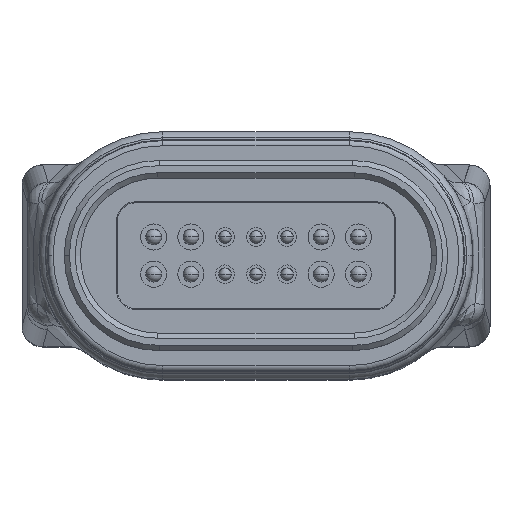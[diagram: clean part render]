
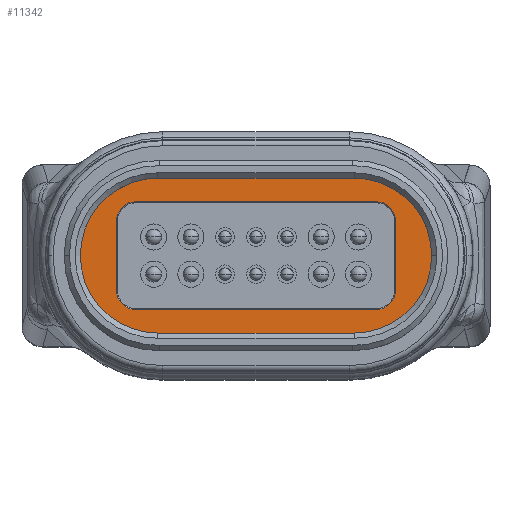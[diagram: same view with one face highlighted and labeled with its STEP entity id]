
A CAD part, top view. The second image highlights one B-rep face of the part: STEP entity #11342.
In plain terms, the highlighted planar face has unit normal (0, 0, 1).
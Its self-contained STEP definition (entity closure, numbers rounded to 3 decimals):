
#337 = ORIENTED_EDGE ( 'NONE', *, *, #929, .T. ) ;
#457 = DIRECTION ( 'NONE',  ( 1., 0., 0. ) ) ;
#584 = DIRECTION ( 'NONE',  ( 1., 0., 0. ) ) ;
#798 = DIRECTION ( 'NONE',  ( -1., 0., 0. ) ) ;
#880 = CIRCLE ( 'NONE', #7388, 0.9 ) ;
#891 = EDGE_CURVE ( 'NONE', #6130, #6328, #986, .T. ) ;
#905 = DIRECTION ( 'NONE',  ( 1., 0., 0. ) ) ;
#929 = EDGE_CURVE ( 'NONE', #8517, #8174, #2845, .T. ) ;
#960 = CARTESIAN_POINT ( 'NONE',  ( -4.75, 0., 1.33 ) ) ;
#986 = CIRCLE ( 'NONE', #6755, 0.9 ) ;
#1099 = LINE ( 'NONE', #6674, #7560 ) ;
#1101 = AXIS2_PLACEMENT_3D ( 'NONE', #8511, #11177, #1482 ) ;
#1262 = VERTEX_POINT ( 'NONE', #10254 ) ;
#1268 = CARTESIAN_POINT ( 'NONE',  ( 8.5, 0., 1.33 ) ) ;
#1289 = VERTEX_POINT ( 'NONE', #2286 ) ;
#1475 = VECTOR ( 'NONE', #11122, 1000. ) ;
#1482 = DIRECTION ( 'NONE',  ( 1., 0., 0. ) ) ;
#1510 = CARTESIAN_POINT ( 'NONE',  ( 4.75, 3.75, 1.33 ) ) ;
#1829 = CARTESIAN_POINT ( 'NONE',  ( -4.75, -3.75, 1.33 ) ) ;
#1927 = EDGE_LOOP ( 'NONE', ( #6397, #4510, #5983, #3448, #8428, #6990, #4462, #10403 ) ) ;
#2000 = DIRECTION ( 'NONE',  ( 1., 0., 0. ) ) ;
#2286 = CARTESIAN_POINT ( 'NONE',  ( -4.75, 3.75, 1.33 ) ) ;
#2827 = ORIENTED_EDGE ( 'NONE', *, *, #10840, .T. ) ;
#2845 = CIRCLE ( 'NONE', #10656, 3.75 ) ;
#2959 = CARTESIAN_POINT ( 'NONE',  ( 6.74, 1.7, 1.33 ) ) ;
#3016 = DIRECTION ( 'NONE',  ( 0., 0., -1. ) ) ;
#3277 = CIRCLE ( 'NONE', #6056, 0.9 ) ;
#3384 = CARTESIAN_POINT ( 'NONE',  ( -5.84, -2.6, 1.33 ) ) ;
#3448 = ORIENTED_EDGE ( 'NONE', *, *, #10071, .T. ) ;
#3636 = VERTEX_POINT ( 'NONE', #7637 ) ;
#3663 = DIRECTION ( 'NONE',  ( 1., 0., 0. ) ) ;
#3825 = CARTESIAN_POINT ( 'NONE',  ( -5.84, 1.7, 1.33 ) ) ;
#3952 = VERTEX_POINT ( 'NONE', #8845 ) ;
#3994 = EDGE_CURVE ( 'NONE', #6328, #1262, #6382, .T. ) ;
#4073 = CARTESIAN_POINT ( 'NONE',  ( -4.75, 0., 1.33 ) ) ;
#4307 = LINE ( 'NONE', #7809, #9484 ) ;
#4367 = CARTESIAN_POINT ( 'NONE',  ( -5.84, -1.7, 1.33 ) ) ;
#4462 = ORIENTED_EDGE ( 'NONE', *, *, #6018, .T. ) ;
#4510 = ORIENTED_EDGE ( 'NONE', *, *, #3994, .T. ) ;
#4512 = VERTEX_POINT ( 'NONE', #2959 ) ;
#4782 = DIRECTION ( 'NONE',  ( 0., 1., 0. ) ) ;
#4979 = LINE ( 'NONE', #7593, #1475 ) ;
#5483 = VECTOR ( 'NONE', #3663, 1000. ) ;
#5619 = CARTESIAN_POINT ( 'NONE',  ( 5.84, -2.6, 1.33 ) ) ;
#5669 = EDGE_LOOP ( 'NONE', ( #2827, #10666, #337, #8271, #11357 ) ) ;
#5828 = PLANE ( 'NONE',  #10617 ) ;
#5877 = CARTESIAN_POINT ( 'NONE',  ( 4.75, 0., 1.33 ) ) ;
#5983 = ORIENTED_EDGE ( 'NONE', *, *, #9795, .T. ) ;
#5993 = FACE_OUTER_BOUND ( 'NONE', #5669, .T. ) ;
#6003 = DIRECTION ( 'NONE',  ( 1., 0., 0. ) ) ;
#6018 = EDGE_CURVE ( 'NONE', #8623, #3636, #880, .T. ) ;
#6056 = AXIS2_PLACEMENT_3D ( 'NONE', #9978, #8291, #2000 ) ;
#6130 = VERTEX_POINT ( 'NONE', #7276 ) ;
#6328 = VERTEX_POINT ( 'NONE', #8112 ) ;
#6382 = LINE ( 'NONE', #7400, #5483 ) ;
#6397 = ORIENTED_EDGE ( 'NONE', *, *, #891, .T. ) ;
#6674 = CARTESIAN_POINT ( 'NONE',  ( -4.75, 3.75, 1.33 ) ) ;
#6682 = FACE_BOUND ( 'NONE', #1927, .T. ) ;
#6694 = DIRECTION ( 'NONE',  ( 0., -1., 0. ) ) ;
#6755 = AXIS2_PLACEMENT_3D ( 'NONE', #3825, #3016, #457 ) ;
#6887 = EDGE_CURVE ( 'NONE', #3636, #6130, #7290, .T. ) ;
#6904 = DIRECTION ( 'NONE',  ( 1., 0., 0. ) ) ;
#6990 = ORIENTED_EDGE ( 'NONE', *, *, #8097, .T. ) ;
#7178 = EDGE_CURVE ( 'NONE', #3952, #10904, #3277, .T. ) ;
#7194 = VECTOR ( 'NONE', #798, 1000. ) ;
#7276 = CARTESIAN_POINT ( 'NONE',  ( -6.74, 1.7, 1.33 ) ) ;
#7290 = LINE ( 'NONE', #9019, #8653 ) ;
#7388 = AXIS2_PLACEMENT_3D ( 'NONE', #4367, #8621, #6003 ) ;
#7400 = CARTESIAN_POINT ( 'NONE',  ( 5.84, 2.6, 1.33 ) ) ;
#7560 = VECTOR ( 'NONE', #11039, 1000. ) ;
#7593 = CARTESIAN_POINT ( 'NONE',  ( -4.75, -3.75, 1.33 ) ) ;
#7637 = CARTESIAN_POINT ( 'NONE',  ( -6.74, -1.7, 1.33 ) ) ;
#7765 = EDGE_CURVE ( 'NONE', #7842, #1289, #1099, .T. ) ;
#7809 = CARTESIAN_POINT ( 'NONE',  ( 6.74, -1.7, 1.33 ) ) ;
#7842 = VERTEX_POINT ( 'NONE', #1510 ) ;
#7907 = EDGE_CURVE ( 'NONE', #8174, #7842, #8475, .T. ) ;
#8097 = EDGE_CURVE ( 'NONE', #10904, #8623, #9639, .T. ) ;
#8112 = CARTESIAN_POINT ( 'NONE',  ( -5.84, 2.6, 1.33 ) ) ;
#8174 = VERTEX_POINT ( 'NONE', #1268 ) ;
#8271 = ORIENTED_EDGE ( 'NONE', *, *, #7907, .T. ) ;
#8291 = DIRECTION ( 'NONE',  ( 0., 0., -1. ) ) ;
#8428 = ORIENTED_EDGE ( 'NONE', *, *, #7178, .T. ) ;
#8472 = CARTESIAN_POINT ( 'NONE',  ( 4.75, 0., 1.33 ) ) ;
#8475 = CIRCLE ( 'NONE', #11251, 3.75 ) ;
#8511 = CARTESIAN_POINT ( 'NONE',  ( 5.84, 1.7, 1.33 ) ) ;
#8517 = VERTEX_POINT ( 'NONE', #10190 ) ;
#8621 = DIRECTION ( 'NONE',  ( 0., 0., -1. ) ) ;
#8623 = VERTEX_POINT ( 'NONE', #3384 ) ;
#8653 = VECTOR ( 'NONE', #4782, 1000. ) ;
#8768 = CARTESIAN_POINT ( 'NONE',  ( -5.84, -2.6, 1.33 ) ) ;
#8845 = CARTESIAN_POINT ( 'NONE',  ( 6.74, -1.7, 1.33 ) ) ;
#8868 = DIRECTION ( 'NONE',  ( 0., 0., 1. ) ) ;
#9019 = CARTESIAN_POINT ( 'NONE',  ( -6.74, 1.7, 1.33 ) ) ;
#9242 = EDGE_CURVE ( 'NONE', #10829, #8517, #4979, .T. ) ;
#9301 = AXIS2_PLACEMENT_3D ( 'NONE', #960, #8868, #905 ) ;
#9363 = DIRECTION ( 'NONE',  ( 1., 0., 0. ) ) ;
#9484 = VECTOR ( 'NONE', #6694, 1000. ) ;
#9494 = CIRCLE ( 'NONE', #9301, 3.75 ) ;
#9588 = DIRECTION ( 'NONE',  ( 0., 0., 1. ) ) ;
#9639 = LINE ( 'NONE', #8768, #7194 ) ;
#9795 = EDGE_CURVE ( 'NONE', #1262, #4512, #11299, .T. ) ;
#9978 = CARTESIAN_POINT ( 'NONE',  ( 5.84, -1.7, 1.33 ) ) ;
#10071 = EDGE_CURVE ( 'NONE', #4512, #3952, #4307, .T. ) ;
#10190 = CARTESIAN_POINT ( 'NONE',  ( 4.75, -3.75, 1.33 ) ) ;
#10254 = CARTESIAN_POINT ( 'NONE',  ( 5.84, 2.6, 1.33 ) ) ;
#10332 = DIRECTION ( 'NONE',  ( 0., 0., 1. ) ) ;
#10340 = DIRECTION ( 'NONE',  ( 0., 0., 1. ) ) ;
#10403 = ORIENTED_EDGE ( 'NONE', *, *, #6887, .T. ) ;
#10617 = AXIS2_PLACEMENT_3D ( 'NONE', #4073, #9588, #9363 ) ;
#10656 = AXIS2_PLACEMENT_3D ( 'NONE', #8472, #10332, #6904 ) ;
#10666 = ORIENTED_EDGE ( 'NONE', *, *, #9242, .T. ) ;
#10829 = VERTEX_POINT ( 'NONE', #1829 ) ;
#10840 = EDGE_CURVE ( 'NONE', #1289, #10829, #9494, .T. ) ;
#10904 = VERTEX_POINT ( 'NONE', #5619 ) ;
#11039 = DIRECTION ( 'NONE',  ( -1., 0., 0. ) ) ;
#11122 = DIRECTION ( 'NONE',  ( 1., 0., 0. ) ) ;
#11177 = DIRECTION ( 'NONE',  ( 0., 0., -1. ) ) ;
#11251 = AXIS2_PLACEMENT_3D ( 'NONE', #5877, #10340, #584 ) ;
#11299 = CIRCLE ( 'NONE', #1101, 0.9 ) ;
#11342 = ADVANCED_FACE ( 'NONE', ( #6682, #5993 ), #5828, .T. ) ;
#11357 = ORIENTED_EDGE ( 'NONE', *, *, #7765, .T. ) ;
